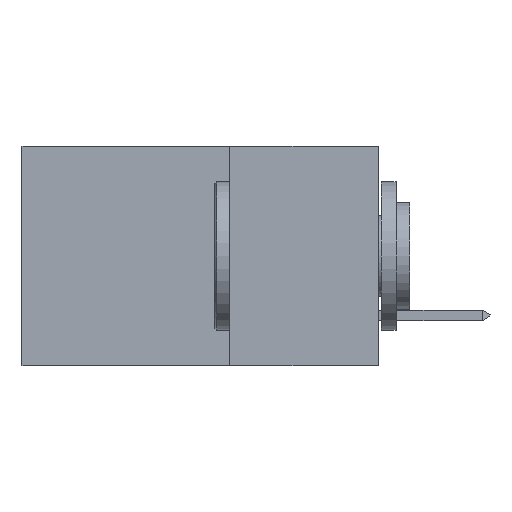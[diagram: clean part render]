
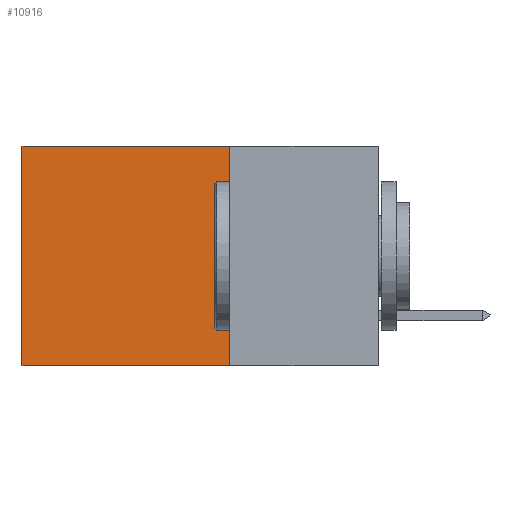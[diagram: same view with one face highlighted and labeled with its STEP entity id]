
A CAD part, left-side view. The second image highlights one B-rep face of the part: STEP entity #10916.
In plain terms, the highlighted planar face has unit normal (-1, 0, 0).
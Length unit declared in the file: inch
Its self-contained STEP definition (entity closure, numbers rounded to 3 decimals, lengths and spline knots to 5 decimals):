
#469 = DIRECTION ( 'NONE',  ( 0., 1., 0. ) ) ;
#963 = EDGE_CURVE ( 'NONE', #6581, #9939, #4651, .T. ) ;
#1088 = EDGE_CURVE ( 'NONE', #9819, #9939, #5806, .T. ) ;
#1091 = VECTOR ( 'NONE', #1662, 39.37008 ) ;
#1597 = CARTESIAN_POINT ( 'NONE',  ( 0.298, 0.6, 0. ) ) ;
#1662 = DIRECTION ( 'NONE',  ( 0., 1., 0. ) ) ;
#1877 = CARTESIAN_POINT ( 'NONE',  ( 0.298, 0.25, 0. ) ) ;
#2332 = LINE ( 'NONE', #4469, #1091 ) ;
#2447 = VERTEX_POINT ( 'NONE', #1877 ) ;
#3453 = DIRECTION ( 'NONE',  ( 0., 0., -1. ) ) ;
#3499 = DIRECTION ( 'NONE',  ( 1., 0., 0. ) ) ;
#3538 = CARTESIAN_POINT ( 'NONE',  ( 0.298, 0.25, -0.37 ) ) ;
#4303 = PLANE ( 'NONE',  #10304 ) ;
#4469 = CARTESIAN_POINT ( 'NONE',  ( 0.298, 0.25, 0. ) ) ;
#4651 = LINE ( 'NONE', #11024, #9914 ) ;
#4830 = ORIENTED_EDGE ( 'NONE', *, *, #6084, .T. ) ;
#5131 = CARTESIAN_POINT ( 'NONE',  ( 0.298, 0.25, 0. ) ) ;
#5251 = VECTOR ( 'NONE', #3453, 39.37008 ) ;
#5263 = DIRECTION ( 'NONE',  ( 0., 0., -1. ) ) ;
#5773 = FACE_OUTER_BOUND ( 'NONE', #10914, .T. ) ;
#5806 = LINE ( 'NONE', #1597, #5251 ) ;
#6084 = EDGE_CURVE ( 'NONE', #2447, #9819, #2332, .T. ) ;
#6368 = VECTOR ( 'NONE', #7906, 39.37008 ) ;
#6581 = VERTEX_POINT ( 'NONE', #3538 ) ;
#7180 = ORIENTED_EDGE ( 'NONE', *, *, #963, .F. ) ;
#7203 = EDGE_CURVE ( 'NONE', #2447, #6581, #8708, .T. ) ;
#7508 = ORIENTED_EDGE ( 'NONE', *, *, #7203, .F. ) ;
#7906 = DIRECTION ( 'NONE',  ( 0., 0., -1. ) ) ;
#7953 = CARTESIAN_POINT ( 'NONE',  ( 0.298, 0.25, 0. ) ) ;
#8662 = ORIENTED_EDGE ( 'NONE', *, *, #1088, .T. ) ;
#8708 = LINE ( 'NONE', #5131, #6368 ) ;
#9819 = VERTEX_POINT ( 'NONE', #11584 ) ;
#9914 = VECTOR ( 'NONE', #469, 39.37008 ) ;
#9939 = VERTEX_POINT ( 'NONE', #10553 ) ;
#10304 = AXIS2_PLACEMENT_3D ( 'NONE', #7953, #3499, #5263 ) ;
#10553 = CARTESIAN_POINT ( 'NONE',  ( 0.298, 0.6, -0.37 ) ) ;
#10914 = EDGE_LOOP ( 'NONE', ( #8662, #7180, #7508, #4830 ) ) ;
#10916 = ADVANCED_FACE ( 'NONE', ( #5773 ), #4303, .F. ) ;
#11024 = CARTESIAN_POINT ( 'NONE',  ( 0.298, 0.25, -0.37 ) ) ;
#11584 = CARTESIAN_POINT ( 'NONE',  ( 0.298, 0.6, 0. ) ) ;
